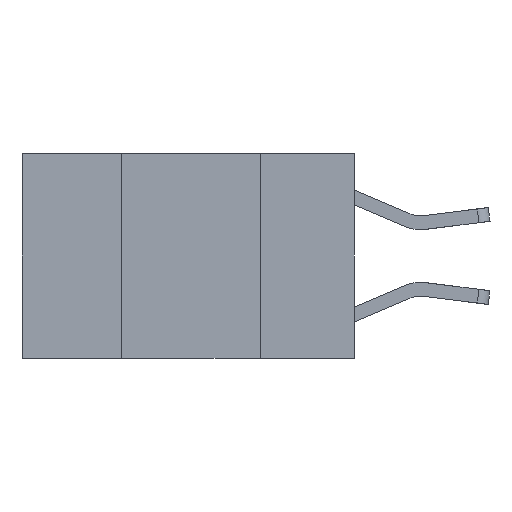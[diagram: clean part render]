
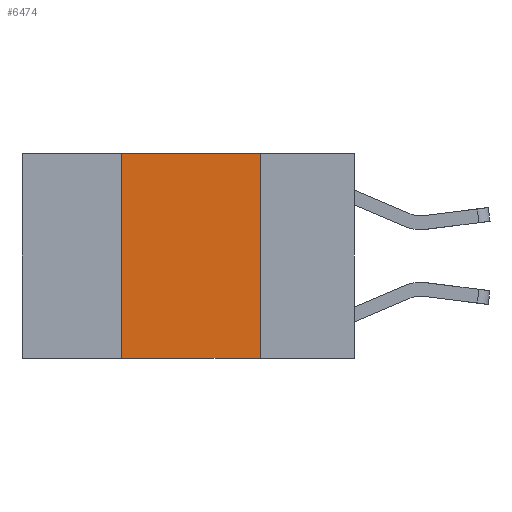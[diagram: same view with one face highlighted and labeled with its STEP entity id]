
A CAD part, left-side view. The second image highlights one B-rep face of the part: STEP entity #6474.
In plain terms, the highlighted planar face has unit normal (-1, 0, 0).
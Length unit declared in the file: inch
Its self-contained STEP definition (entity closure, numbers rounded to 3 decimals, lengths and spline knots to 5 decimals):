
#69 = VERTEX_POINT ( 'NONE', #2943 ) ;
#260 = CARTESIAN_POINT ( 'NONE',  ( 0., 0.42, -0.37 ) ) ;
#834 = ORIENTED_EDGE ( 'NONE', *, *, #6124, .F. ) ;
#863 = VERTEX_POINT ( 'NONE', #5837 ) ;
#1111 = EDGE_CURVE ( 'NONE', #2846, #863, #1360, .T. ) ;
#1177 = CARTESIAN_POINT ( 'NONE',  ( 0., 0.6, 0. ) ) ;
#1261 = DIRECTION ( 'NONE',  ( 0., 0., -1. ) ) ;
#1311 = DIRECTION ( 'NONE',  ( 1., 0., 0. ) ) ;
#1360 = LINE ( 'NONE', #3430, #6094 ) ;
#2357 = DIRECTION ( 'NONE',  ( 0., -1., 0. ) ) ;
#2474 = CARTESIAN_POINT ( 'NONE',  ( 0., 0.42, 0. ) ) ;
#2846 = VERTEX_POINT ( 'NONE', #2474 ) ;
#2943 = CARTESIAN_POINT ( 'NONE',  ( 0., 0.17, -0.37 ) ) ;
#3430 = CARTESIAN_POINT ( 'NONE',  ( 0., 0.6, 0. ) ) ;
#3881 = VERTEX_POINT ( 'NONE', #260 ) ;
#3993 = LINE ( 'NONE', #6756, #9090 ) ;
#4075 = ORIENTED_EDGE ( 'NONE', *, *, #8046, .T. ) ;
#4159 = ORIENTED_EDGE ( 'NONE', *, *, #1111, .F. ) ;
#4603 = VECTOR ( 'NONE', #2357, 39.37008 ) ;
#5024 = DIRECTION ( 'NONE',  ( 0., -1., 0. ) ) ;
#5116 = EDGE_CURVE ( 'NONE', #3881, #2846, #3993, .T. ) ;
#5726 = DIRECTION ( 'NONE',  ( 0., 0., -1. ) ) ;
#5837 = CARTESIAN_POINT ( 'NONE',  ( 0., 0.17, 0. ) ) ;
#5989 = CARTESIAN_POINT ( 'NONE',  ( 0., 0.6, -0.37 ) ) ;
#6094 = VECTOR ( 'NONE', #5024, 39.37008 ) ;
#6124 = EDGE_CURVE ( 'NONE', #863, #69, #6551, .T. ) ;
#6136 = PLANE ( 'NONE',  #7366 ) ;
#6239 = ORIENTED_EDGE ( 'NONE', *, *, #5116, .F. ) ;
#6269 = DIRECTION ( 'NONE',  ( 0., 0., 1. ) ) ;
#6474 = ADVANCED_FACE ( 'NONE', ( #7491 ), #6136, .F. ) ;
#6551 = LINE ( 'NONE', #8489, #9002 ) ;
#6756 = CARTESIAN_POINT ( 'NONE',  ( 0., 0.42, 0. ) ) ;
#7366 = AXIS2_PLACEMENT_3D ( 'NONE', #1177, #1311, #1261 ) ;
#7491 = FACE_OUTER_BOUND ( 'NONE', #8684, .T. ) ;
#8046 = EDGE_CURVE ( 'NONE', #3881, #69, #8711, .T. ) ;
#8489 = CARTESIAN_POINT ( 'NONE',  ( 0., 0.17, 0. ) ) ;
#8684 = EDGE_LOOP ( 'NONE', ( #834, #4159, #6239, #4075 ) ) ;
#8711 = LINE ( 'NONE', #5989, #4603 ) ;
#9002 = VECTOR ( 'NONE', #5726, 39.37008 ) ;
#9090 = VECTOR ( 'NONE', #6269, 39.37008 ) ;
